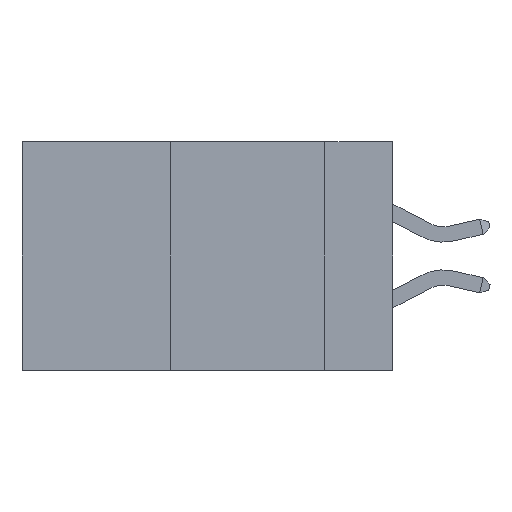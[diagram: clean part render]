
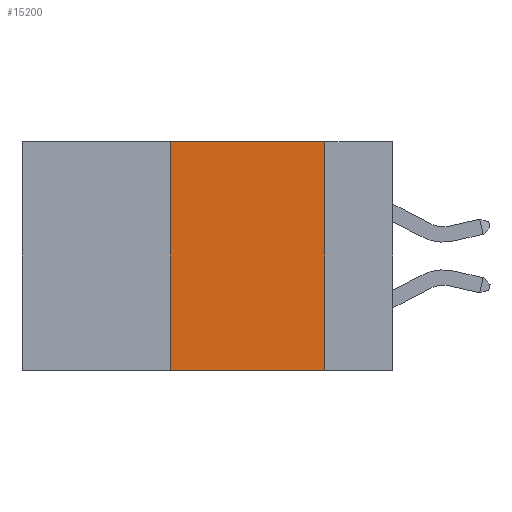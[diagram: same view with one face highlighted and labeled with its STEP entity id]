
A CAD part, left-side view. The second image highlights one B-rep face of the part: STEP entity #15200.
In plain terms, the highlighted planar face has unit normal (-1, 0, 0).
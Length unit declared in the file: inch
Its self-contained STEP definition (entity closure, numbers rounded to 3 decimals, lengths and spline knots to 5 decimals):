
#532 = CARTESIAN_POINT ( 'NONE',  ( 0., 0.6, 0. ) ) ;
#1402 = CARTESIAN_POINT ( 'NONE',  ( 0., 0.11, 0. ) ) ;
#2817 = VERTEX_POINT ( 'NONE', #10295 ) ;
#3208 = VECTOR ( 'NONE', #26176, 39.37008 ) ;
#3663 = LINE ( 'NONE', #29721, #11569 ) ;
#4100 = VERTEX_POINT ( 'NONE', #21888 ) ;
#4517 = EDGE_CURVE ( 'NONE', #2817, #4100, #3663, .T. ) ;
#6161 = EDGE_CURVE ( 'NONE', #2817, #6383, #33631, .T. ) ;
#6383 = VERTEX_POINT ( 'NONE', #34375 ) ;
#8637 = ORIENTED_EDGE ( 'NONE', *, *, #24621, .F. ) ;
#8772 = CARTESIAN_POINT ( 'NONE',  ( 0., 0.6, 0. ) ) ;
#8938 = FACE_OUTER_BOUND ( 'NONE', #13209, .T. ) ;
#10295 = CARTESIAN_POINT ( 'NONE',  ( 0., 0.36, -0.37 ) ) ;
#10408 = VECTOR ( 'NONE', #33289, 39.37008 ) ;
#11569 = VECTOR ( 'NONE', #11834, 39.37008 ) ;
#11834 = DIRECTION ( 'NONE',  ( 0., -1., 0. ) ) ;
#12484 = DIRECTION ( 'NONE',  ( 1., 0., 0. ) ) ;
#13209 = EDGE_LOOP ( 'NONE', ( #8637, #25557, #17968, #27621 ) ) ;
#14038 = DIRECTION ( 'NONE',  ( 0., 0., 1. ) ) ;
#15200 = ADVANCED_FACE ( 'NONE', ( #8938 ), #36485, .F. ) ;
#17616 = AXIS2_PLACEMENT_3D ( 'NONE', #532, #12484, #21730 ) ;
#17823 = EDGE_CURVE ( 'NONE', #6383, #25383, #18034, .T. ) ;
#17968 = ORIENTED_EDGE ( 'NONE', *, *, #6161, .F. ) ;
#18034 = LINE ( 'NONE', #8772, #3208 ) ;
#21376 = CARTESIAN_POINT ( 'NONE',  ( 0., 0.36, 0. ) ) ;
#21431 = CARTESIAN_POINT ( 'NONE',  ( 0., 0.11, 0. ) ) ;
#21730 = DIRECTION ( 'NONE',  ( 0., 0., -1. ) ) ;
#21888 = CARTESIAN_POINT ( 'NONE',  ( 0., 0.11, -0.37 ) ) ;
#24621 = EDGE_CURVE ( 'NONE', #25383, #4100, #35463, .T. ) ;
#25383 = VERTEX_POINT ( 'NONE', #1402 ) ;
#25557 = ORIENTED_EDGE ( 'NONE', *, *, #17823, .F. ) ;
#26176 = DIRECTION ( 'NONE',  ( 0., -1., 0. ) ) ;
#27621 = ORIENTED_EDGE ( 'NONE', *, *, #4517, .T. ) ;
#29721 = CARTESIAN_POINT ( 'NONE',  ( 0., 0.6, -0.37 ) ) ;
#30882 = VECTOR ( 'NONE', #14038, 39.37008 ) ;
#33289 = DIRECTION ( 'NONE',  ( 0., 0., -1. ) ) ;
#33631 = LINE ( 'NONE', #21376, #30882 ) ;
#34375 = CARTESIAN_POINT ( 'NONE',  ( 0., 0.36, 0. ) ) ;
#35463 = LINE ( 'NONE', #21431, #10408 ) ;
#36485 = PLANE ( 'NONE',  #17616 ) ;
